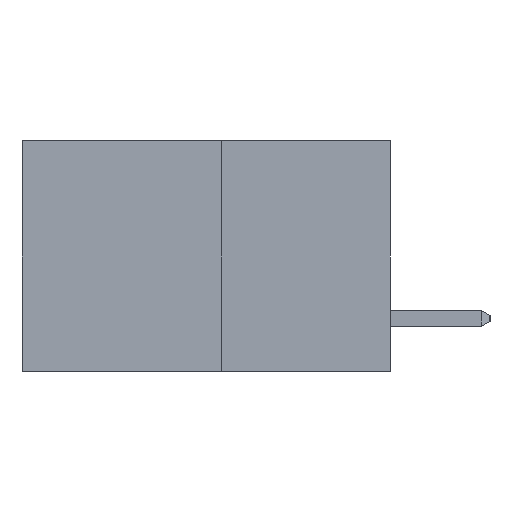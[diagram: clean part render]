
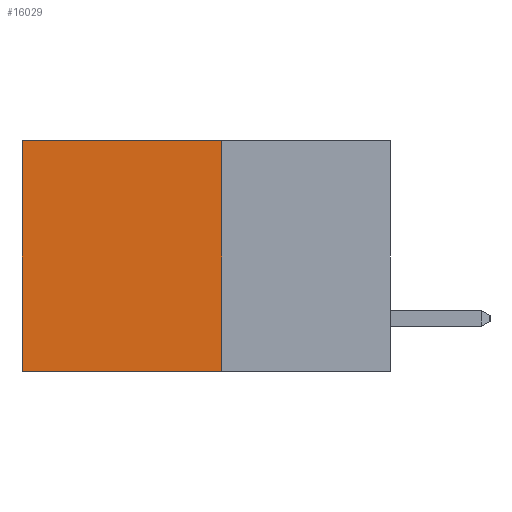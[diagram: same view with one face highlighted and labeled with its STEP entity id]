
A CAD part, left-side view. The second image highlights one B-rep face of the part: STEP entity #16029.
In plain terms, the highlighted planar face has unit normal (-1, 0, 0).
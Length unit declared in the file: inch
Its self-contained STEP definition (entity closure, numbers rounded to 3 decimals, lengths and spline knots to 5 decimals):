
#349 = DIRECTION ( 'NONE',  ( 0., 0., -1. ) ) ;
#437 = VECTOR ( 'NONE', #349, 39.37008 ) ;
#574 = DIRECTION ( 'NONE',  ( 0., 0., -1. ) ) ;
#717 = CARTESIAN_POINT ( 'NONE',  ( 0.277, 0.27, -0.37 ) ) ;
#2162 = VERTEX_POINT ( 'NONE', #15606 ) ;
#2436 = DIRECTION ( 'NONE',  ( 0., 0., -1. ) ) ;
#2926 = EDGE_CURVE ( 'NONE', #11174, #14255, #13317, .T. ) ;
#3049 = AXIS2_PLACEMENT_3D ( 'NONE', #717, #12630, #2436 ) ;
#3687 = CARTESIAN_POINT ( 'NONE',  ( 0.277, 0.27, -0.37 ) ) ;
#5734 = CARTESIAN_POINT ( 'NONE',  ( 0.277, 0.27, -0.37 ) ) ;
#6291 = FACE_OUTER_BOUND ( 'NONE', #16737, .T. ) ;
#7891 = VECTOR ( 'NONE', #17535, 39.37008 ) ;
#7901 = ORIENTED_EDGE ( 'NONE', *, *, #19489, .T. ) ;
#8453 = VERTEX_POINT ( 'NONE', #19672 ) ;
#8668 = DIRECTION ( 'NONE',  ( 0., 1., 0. ) ) ;
#8879 = VECTOR ( 'NONE', #8668, 39.37008 ) ;
#9180 = CARTESIAN_POINT ( 'NONE',  ( 0.277, 0.27, 0. ) ) ;
#9188 = CARTESIAN_POINT ( 'NONE',  ( 0.277, 0.27, -0.37 ) ) ;
#10961 = PLANE ( 'NONE',  #3049 ) ;
#11174 = VERTEX_POINT ( 'NONE', #9188 ) ;
#12366 = LINE ( 'NONE', #9180, #7891 ) ;
#12630 = DIRECTION ( 'NONE',  ( 1., 0., 0. ) ) ;
#12830 = CARTESIAN_POINT ( 'NONE',  ( 0.277, 0.59, -0.37 ) ) ;
#12922 = LINE ( 'NONE', #17252, #437 ) ;
#12972 = EDGE_CURVE ( 'NONE', #2162, #11174, #19183, .T. ) ;
#13317 = LINE ( 'NONE', #3687, #8879 ) ;
#14255 = VERTEX_POINT ( 'NONE', #12830 ) ;
#14296 = VECTOR ( 'NONE', #574, 39.37008 ) ;
#14773 = ORIENTED_EDGE ( 'NONE', *, *, #12972, .F. ) ;
#15205 = ORIENTED_EDGE ( 'NONE', *, *, #2926, .F. ) ;
#15606 = CARTESIAN_POINT ( 'NONE',  ( 0.277, 0.27, 0. ) ) ;
#16029 = ADVANCED_FACE ( 'NONE', ( #6291 ), #10961, .F. ) ;
#16737 = EDGE_LOOP ( 'NONE', ( #18444, #15205, #14773, #7901 ) ) ;
#17252 = CARTESIAN_POINT ( 'NONE',  ( 0.277, 0.59, -0.37 ) ) ;
#17535 = DIRECTION ( 'NONE',  ( 0., 1., 0. ) ) ;
#18444 = ORIENTED_EDGE ( 'NONE', *, *, #18631, .T. ) ;
#18631 = EDGE_CURVE ( 'NONE', #8453, #14255, #12922, .T. ) ;
#19183 = LINE ( 'NONE', #5734, #14296 ) ;
#19489 = EDGE_CURVE ( 'NONE', #2162, #8453, #12366, .T. ) ;
#19672 = CARTESIAN_POINT ( 'NONE',  ( 0.277, 0.59, 0. ) ) ;
